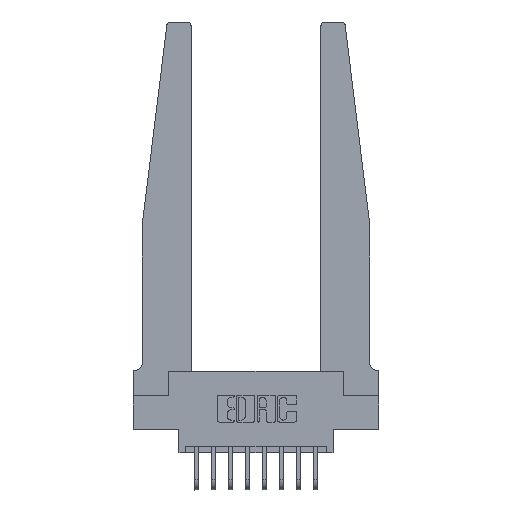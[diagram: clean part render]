
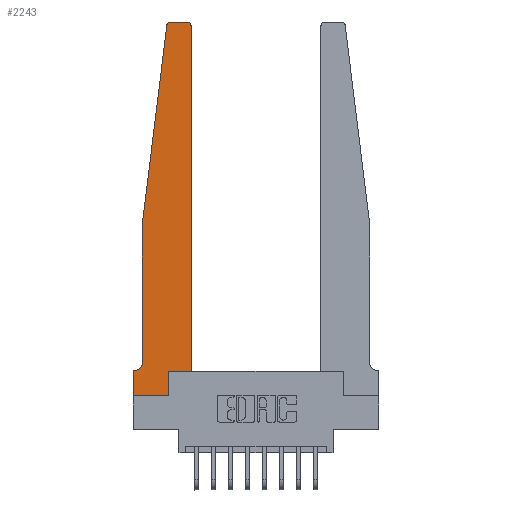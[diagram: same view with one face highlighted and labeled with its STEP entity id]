
A CAD part, top view. The second image highlights one B-rep face of the part: STEP entity #2243.
In plain terms, the highlighted planar face has unit normal (0, 0, 1).
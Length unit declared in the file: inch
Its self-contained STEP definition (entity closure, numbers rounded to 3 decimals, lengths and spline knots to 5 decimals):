
#195 = CARTESIAN_POINT ( 'NONE',  ( 0.395, 2.75, 0.37 ) ) ;
#267 = DIRECTION ( 'NONE',  ( -1., 0., 0. ) ) ;
#323 = CARTESIAN_POINT ( 'NONE',  ( 0.25, 2.75, 0.37 ) ) ;
#397 = VERTEX_POINT ( 'NONE', #7626 ) ;
#547 = CARTESIAN_POINT ( 'NONE',  ( 0.425, 0.18, 0.37 ) ) ;
#556 = CARTESIAN_POINT ( 'NONE',  ( 0.2605, 0.18, 0.37 ) ) ;
#790 = LINE ( 'NONE', #13541, #10657 ) ;
#1050 = LINE ( 'NONE', #11166, #13060 ) ;
#1053 = CARTESIAN_POINT ( 'NONE',  ( 0., 0., 0.37 ) ) ;
#1107 = ORIENTED_EDGE ( 'NONE', *, *, #1288, .T. ) ;
#1147 = ORIENTED_EDGE ( 'NONE', *, *, #4636, .T. ) ;
#1288 = EDGE_CURVE ( 'NONE', #397, #9199, #11637, .T. ) ;
#1623 = CARTESIAN_POINT ( 'NONE',  ( 0.065, 1.25, 0.37 ) ) ;
#1726 = EDGE_LOOP ( 'NONE', ( #2813, #11069, #5795, #9590, #4652, #9192, #3567, #12435, #8510, #1147, #6253, #1107 ) ) ;
#1818 = CARTESIAN_POINT ( 'NONE',  ( 0., 0.1875, 0.37 ) ) ;
#2038 = DIRECTION ( 'NONE',  ( 1., 0., 0. ) ) ;
#2109 = LINE ( 'NONE', #1053, #4651 ) ;
#2229 = EDGE_CURVE ( 'NONE', #9967, #12639, #10959, .T. ) ;
#2243 = ADVANCED_FACE ( 'NONE', ( #3027 ), #12227, .T. ) ;
#2253 = DIRECTION ( 'NONE',  ( 1., 0., 0. ) ) ;
#2262 = LINE ( 'NONE', #323, #9978 ) ;
#2503 = LINE ( 'NONE', #10645, #7610 ) ;
#2813 = ORIENTED_EDGE ( 'NONE', *, *, #4565, .T. ) ;
#2825 = VERTEX_POINT ( 'NONE', #3347 ) ;
#2936 = DIRECTION ( 'NONE',  ( 1., 0., 0. ) ) ;
#3027 = FACE_OUTER_BOUND ( 'NONE', #1726, .T. ) ;
#3268 = CARTESIAN_POINT ( 'NONE',  ( 0.065, 0.2375, 0.37 ) ) ;
#3347 = CARTESIAN_POINT ( 'NONE',  ( 0.425, 0.18, 0.37 ) ) ;
#3567 = ORIENTED_EDGE ( 'NONE', *, *, #12029, .T. ) ;
#3599 = CARTESIAN_POINT ( 'NONE',  ( 0.27653, 2.75, 0.37 ) ) ;
#3766 = VERTEX_POINT ( 'NONE', #3599 ) ;
#3985 = AXIS2_PLACEMENT_3D ( 'NONE', #14496, #6149, #6370 ) ;
#4106 = CARTESIAN_POINT ( 'NONE',  ( 0., 0., 0.37 ) ) ;
#4129 = DIRECTION ( 'NONE',  ( 0., 0., 1. ) ) ;
#4565 = EDGE_CURVE ( 'NONE', #9199, #3766, #2262, .T. ) ;
#4636 = EDGE_CURVE ( 'NONE', #12639, #2825, #7575, .T. ) ;
#4651 = VECTOR ( 'NONE', #2253, 39.37008 ) ;
#4652 = ORIENTED_EDGE ( 'NONE', *, *, #6828, .T. ) ;
#5306 = CARTESIAN_POINT ( 'NONE',  ( 0.2605, 0.18, 0.37 ) ) ;
#5344 = EDGE_CURVE ( 'NONE', #3766, #9336, #11677, .T. ) ;
#5795 = ORIENTED_EDGE ( 'NONE', *, *, #8670, .T. ) ;
#6118 = VECTOR ( 'NONE', #14634, 39.37008 ) ;
#6149 = DIRECTION ( 'NONE',  ( 0., 0., -1. ) ) ;
#6168 = EDGE_CURVE ( 'NONE', #7446, #10135, #2503, .T. ) ;
#6253 = ORIENTED_EDGE ( 'NONE', *, *, #9812, .T. ) ;
#6370 = DIRECTION ( 'NONE',  ( -1., 0., 0. ) ) ;
#6380 = DIRECTION ( 'NONE',  ( -0.122, -0.992, 0. ) ) ;
#6430 = DIRECTION ( 'NONE',  ( 0., 0., 1. ) ) ;
#6781 = AXIS2_PLACEMENT_3D ( 'NONE', #11388, #13787, #2038 ) ;
#6828 = EDGE_CURVE ( 'NONE', #9458, #7446, #8605, .T. ) ;
#7117 = DIRECTION ( 'NONE',  ( -1., 0., 0. ) ) ;
#7156 = AXIS2_PLACEMENT_3D ( 'NONE', #1818, #6430, #8039 ) ;
#7225 = CARTESIAN_POINT ( 'NONE',  ( 0., 0., 0.37 ) ) ;
#7446 = VERTEX_POINT ( 'NONE', #10826 ) ;
#7575 = LINE ( 'NONE', #547, #12408 ) ;
#7610 = VECTOR ( 'NONE', #267, 39.37008 ) ;
#7626 = CARTESIAN_POINT ( 'NONE',  ( 0.425, 2.72, 0.37 ) ) ;
#7999 = CARTESIAN_POINT ( 'NONE',  ( 0.065, 1.25, 0.37 ) ) ;
#8039 = DIRECTION ( 'NONE',  ( 1., 0., 0. ) ) ;
#8510 = ORIENTED_EDGE ( 'NONE', *, *, #2229, .T. ) ;
#8605 = CIRCLE ( 'NONE', #3985, 0.05 ) ;
#8663 = DIRECTION ( 'NONE',  ( 0., 1., 0. ) ) ;
#8670 = EDGE_CURVE ( 'NONE', #9336, #10325, #790, .T. ) ;
#8769 = DIRECTION ( 'NONE',  ( 1., 0., 0. ) ) ;
#8841 = CARTESIAN_POINT ( 'NONE',  ( 0.27653, 2.72, 0.37 ) ) ;
#9192 = ORIENTED_EDGE ( 'NONE', *, *, #6168, .T. ) ;
#9199 = VERTEX_POINT ( 'NONE', #195 ) ;
#9336 = VERTEX_POINT ( 'NONE', #12170 ) ;
#9458 = VERTEX_POINT ( 'NONE', #3268 ) ;
#9590 = ORIENTED_EDGE ( 'NONE', *, *, #13676, .T. ) ;
#9690 = VECTOR ( 'NONE', #11878, 39.37008 ) ;
#9812 = EDGE_CURVE ( 'NONE', #2825, #397, #1050, .T. ) ;
#9967 = VERTEX_POINT ( 'NONE', #12051 ) ;
#9978 = VECTOR ( 'NONE', #7117, 39.37008 ) ;
#10013 = LINE ( 'NONE', #1623, #6118 ) ;
#10135 = VERTEX_POINT ( 'NONE', #11201 ) ;
#10325 = VERTEX_POINT ( 'NONE', #7999 ) ;
#10645 = CARTESIAN_POINT ( 'NONE',  ( 0.065, 0.1875, 0.37 ) ) ;
#10657 = VECTOR ( 'NONE', #6380, 39.37008 ) ;
#10826 = CARTESIAN_POINT ( 'NONE',  ( 0.015, 0.1875, 0.37 ) ) ;
#10959 = LINE ( 'NONE', #5306, #13928 ) ;
#11069 = ORIENTED_EDGE ( 'NONE', *, *, #5344, .T. ) ;
#11166 = CARTESIAN_POINT ( 'NONE',  ( 0.425, 0.18, 0.37 ) ) ;
#11201 = CARTESIAN_POINT ( 'NONE',  ( 0., 0.1875, 0.37 ) ) ;
#11388 = CARTESIAN_POINT ( 'NONE',  ( 0.395, 2.72, 0.37 ) ) ;
#11637 = CIRCLE ( 'NONE', #6781, 0.03 ) ;
#11677 = CIRCLE ( 'NONE', #13616, 0.03 ) ;
#11878 = DIRECTION ( 'NONE',  ( 0., -1., 0. ) ) ;
#12029 = EDGE_CURVE ( 'NONE', #10135, #12200, #12035, .T. ) ;
#12035 = LINE ( 'NONE', #7225, #9690 ) ;
#12051 = CARTESIAN_POINT ( 'NONE',  ( 0.2605, 0., 0.37 ) ) ;
#12170 = CARTESIAN_POINT ( 'NONE',  ( 0.24675, 2.72367, 0.37 ) ) ;
#12200 = VERTEX_POINT ( 'NONE', #4106 ) ;
#12227 = PLANE ( 'NONE',  #7156 ) ;
#12408 = VECTOR ( 'NONE', #2936, 39.37008 ) ;
#12435 = ORIENTED_EDGE ( 'NONE', *, *, #12724, .T. ) ;
#12639 = VERTEX_POINT ( 'NONE', #556 ) ;
#12724 = EDGE_CURVE ( 'NONE', #12200, #9967, #2109, .T. ) ;
#13060 = VECTOR ( 'NONE', #13647, 39.37008 ) ;
#13541 = CARTESIAN_POINT ( 'NONE',  ( 0.065, 1.25, 0.37 ) ) ;
#13616 = AXIS2_PLACEMENT_3D ( 'NONE', #8841, #4129, #8769 ) ;
#13647 = DIRECTION ( 'NONE',  ( 0., 1., 0. ) ) ;
#13676 = EDGE_CURVE ( 'NONE', #10325, #9458, #10013, .T. ) ;
#13787 = DIRECTION ( 'NONE',  ( 0., 0., 1. ) ) ;
#13928 = VECTOR ( 'NONE', #8663, 39.37008 ) ;
#14496 = CARTESIAN_POINT ( 'NONE',  ( 0.015, 0.2375, 0.37 ) ) ;
#14634 = DIRECTION ( 'NONE',  ( 0., -1., 0. ) ) ;
